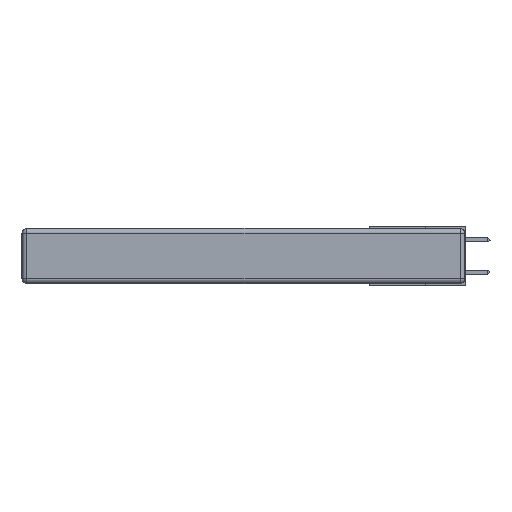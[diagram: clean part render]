
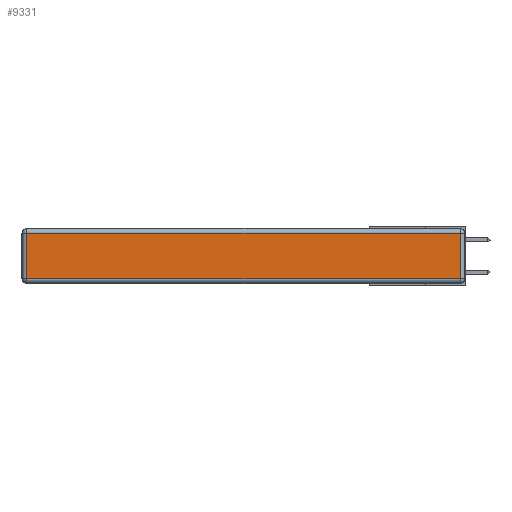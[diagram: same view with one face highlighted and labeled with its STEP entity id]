
A CAD part, left-side view. The second image highlights one B-rep face of the part: STEP entity #9331.
In plain terms, the highlighted planar face has unit normal (-1, 0, 0).
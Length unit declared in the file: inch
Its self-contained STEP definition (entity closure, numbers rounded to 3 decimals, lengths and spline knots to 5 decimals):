
#407 = VECTOR ( 'NONE', #5384, 39.37008 ) ;
#465 = FACE_OUTER_BOUND ( 'NONE', #14634, .T. ) ;
#724 = CARTESIAN_POINT ( 'NONE',  ( 0., 0.03, -0.343 ) ) ;
#2162 = LINE ( 'NONE', #724, #16576 ) ;
#2873 = CARTESIAN_POINT ( 'NONE',  ( 0., 2.72, -0.03 ) ) ;
#3148 = DIRECTION ( 'NONE',  ( 0., 1., 0. ) ) ;
#3457 = LINE ( 'NONE', #27680, #407 ) ;
#5384 = DIRECTION ( 'NONE',  ( 0., 0., -1. ) ) ;
#5841 = DIRECTION ( 'NONE',  ( 0., 0., 1. ) ) ;
#7530 = CARTESIAN_POINT ( 'NONE',  ( 0., 2.75, -0.03 ) ) ;
#9331 = ADVANCED_FACE ( 'NONE', ( #465 ), #11843, .T. ) ;
#10335 = DIRECTION ( 'NONE',  ( 0., -1., 0. ) ) ;
#11843 = PLANE ( 'NONE',  #23405 ) ;
#12240 = ORIENTED_EDGE ( 'NONE', *, *, #26143, .T. ) ;
#12375 = LINE ( 'NONE', #7530, #26056 ) ;
#12704 = ORIENTED_EDGE ( 'NONE', *, *, #15384, .T. ) ;
#14634 = EDGE_LOOP ( 'NONE', ( #26449, #15111, #12240, #12704 ) ) ;
#15111 = ORIENTED_EDGE ( 'NONE', *, *, #17334, .T. ) ;
#15384 = EDGE_CURVE ( 'NONE', #25858, #25023, #3457, .T. ) ;
#16380 = CARTESIAN_POINT ( 'NONE',  ( 0., 0., -0.343 ) ) ;
#16576 = VECTOR ( 'NONE', #5841, 39.37008 ) ;
#16580 = CARTESIAN_POINT ( 'NONE',  ( 0., 2.72, -0.313 ) ) ;
#17334 = EDGE_CURVE ( 'NONE', #22042, #22027, #2162, .T. ) ;
#18413 = VECTOR ( 'NONE', #10335, 39.37008 ) ;
#18970 = CARTESIAN_POINT ( 'NONE',  ( 0., 0.03, -0.03 ) ) ;
#19315 = EDGE_CURVE ( 'NONE', #25023, #22042, #28700, .T. ) ;
#19389 = CARTESIAN_POINT ( 'NONE',  ( 0., 0.03, -0.313 ) ) ;
#22027 = VERTEX_POINT ( 'NONE', #18970 ) ;
#22042 = VERTEX_POINT ( 'NONE', #19389 ) ;
#23405 = AXIS2_PLACEMENT_3D ( 'NONE', #16380, #23929, #23530 ) ;
#23530 = DIRECTION ( 'NONE',  ( 0., 0., 1. ) ) ;
#23929 = DIRECTION ( 'NONE',  ( -1., 0., 0. ) ) ;
#25023 = VERTEX_POINT ( 'NONE', #16580 ) ;
#25858 = VERTEX_POINT ( 'NONE', #2873 ) ;
#26056 = VECTOR ( 'NONE', #3148, 39.37008 ) ;
#26143 = EDGE_CURVE ( 'NONE', #22027, #25858, #12375, .T. ) ;
#26449 = ORIENTED_EDGE ( 'NONE', *, *, #19315, .T. ) ;
#27680 = CARTESIAN_POINT ( 'NONE',  ( 0., 2.72, -0.343 ) ) ;
#28700 = LINE ( 'NONE', #29873, #18413 ) ;
#29873 = CARTESIAN_POINT ( 'NONE',  ( 0., 0., -0.313 ) ) ;
